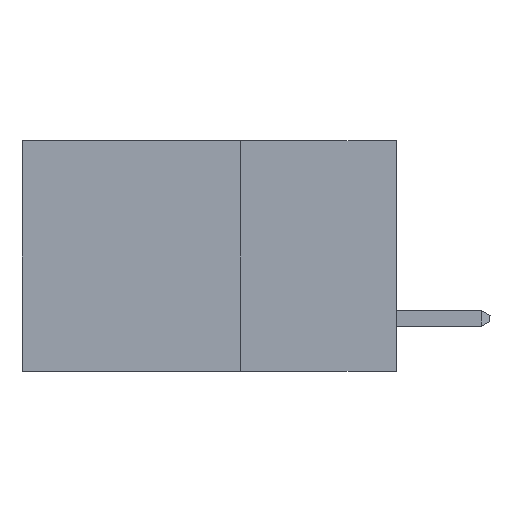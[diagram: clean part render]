
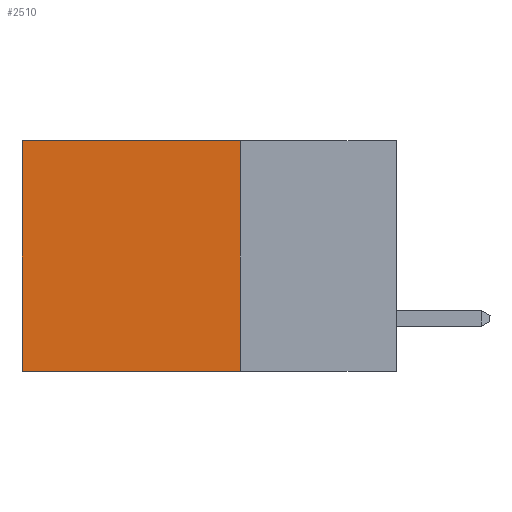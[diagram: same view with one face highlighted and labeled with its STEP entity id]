
A CAD part, left-side view. The second image highlights one B-rep face of the part: STEP entity #2510.
In plain terms, the highlighted planar face has unit normal (-1, 0, 0).
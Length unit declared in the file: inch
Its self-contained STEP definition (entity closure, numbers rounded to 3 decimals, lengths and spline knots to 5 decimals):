
#218 = CARTESIAN_POINT ( 'NONE',  ( 0.2615, 0.6, -0.37 ) ) ;
#584 = LINE ( 'NONE', #218, #20552 ) ;
#1205 = AXIS2_PLACEMENT_3D ( 'NONE', #22574, #20450, #7180 ) ;
#1521 = FACE_OUTER_BOUND ( 'NONE', #10568, .T. ) ;
#2301 = EDGE_CURVE ( 'NONE', #18653, #15253, #584, .T. ) ;
#2510 = ADVANCED_FACE ( 'NONE', ( #1521 ), #24207, .F. ) ;
#4836 = EDGE_CURVE ( 'NONE', #8056, #18653, #14449, .T. ) ;
#6255 = ORIENTED_EDGE ( 'NONE', *, *, #4836, .T. ) ;
#7180 = DIRECTION ( 'NONE',  ( 0., 0., -1. ) ) ;
#7498 = ORIENTED_EDGE ( 'NONE', *, *, #23859, .F. ) ;
#8037 = LINE ( 'NONE', #13213, #14017 ) ;
#8056 = VERTEX_POINT ( 'NONE', #13482 ) ;
#8773 = VECTOR ( 'NONE', #18331, 39.37008 ) ;
#9103 = CARTESIAN_POINT ( 'NONE',  ( 0.2615, 0.6, 0. ) ) ;
#10568 = EDGE_LOOP ( 'NONE', ( #14109, #24155, #7498, #6255 ) ) ;
#12088 = VERTEX_POINT ( 'NONE', #22638 ) ;
#13213 = CARTESIAN_POINT ( 'NONE',  ( 0.2615, 0.25, -0.37 ) ) ;
#13482 = CARTESIAN_POINT ( 'NONE',  ( 0.2615, 0.25, 0. ) ) ;
#14017 = VECTOR ( 'NONE', #20811, 39.37008 ) ;
#14109 = ORIENTED_EDGE ( 'NONE', *, *, #2301, .T. ) ;
#14449 = LINE ( 'NONE', #22318, #8773 ) ;
#15253 = VERTEX_POINT ( 'NONE', #17030 ) ;
#15758 = DIRECTION ( 'NONE',  ( 0., 0., -1. ) ) ;
#16580 = VECTOR ( 'NONE', #24198, 39.37008 ) ;
#17030 = CARTESIAN_POINT ( 'NONE',  ( 0.2615, 0.6, -0.37 ) ) ;
#18067 = EDGE_CURVE ( 'NONE', #12088, #15253, #8037, .T. ) ;
#18331 = DIRECTION ( 'NONE',  ( 0., 1., 0. ) ) ;
#18653 = VERTEX_POINT ( 'NONE', #9103 ) ;
#20329 = CARTESIAN_POINT ( 'NONE',  ( 0.2615, 0.25, -0.37 ) ) ;
#20440 = LINE ( 'NONE', #20329, #16580 ) ;
#20450 = DIRECTION ( 'NONE',  ( 1., 0., 0. ) ) ;
#20552 = VECTOR ( 'NONE', #15758, 39.37008 ) ;
#20811 = DIRECTION ( 'NONE',  ( 0., 1., 0. ) ) ;
#22318 = CARTESIAN_POINT ( 'NONE',  ( 0.2615, 0.25, 0. ) ) ;
#22574 = CARTESIAN_POINT ( 'NONE',  ( 0.2615, 0.25, -0.37 ) ) ;
#22638 = CARTESIAN_POINT ( 'NONE',  ( 0.2615, 0.25, -0.37 ) ) ;
#23859 = EDGE_CURVE ( 'NONE', #8056, #12088, #20440, .T. ) ;
#24155 = ORIENTED_EDGE ( 'NONE', *, *, #18067, .F. ) ;
#24198 = DIRECTION ( 'NONE',  ( 0., 0., -1. ) ) ;
#24207 = PLANE ( 'NONE',  #1205 ) ;
